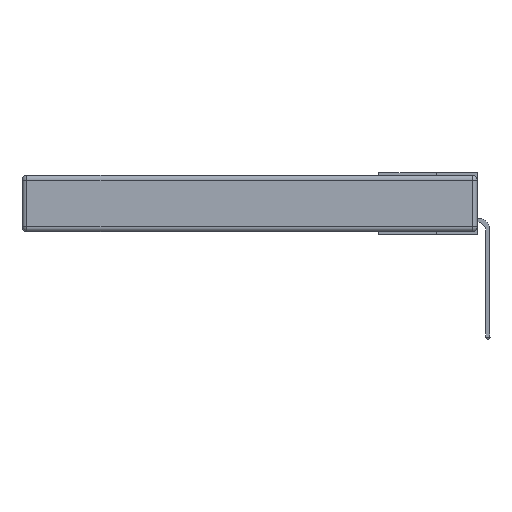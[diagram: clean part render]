
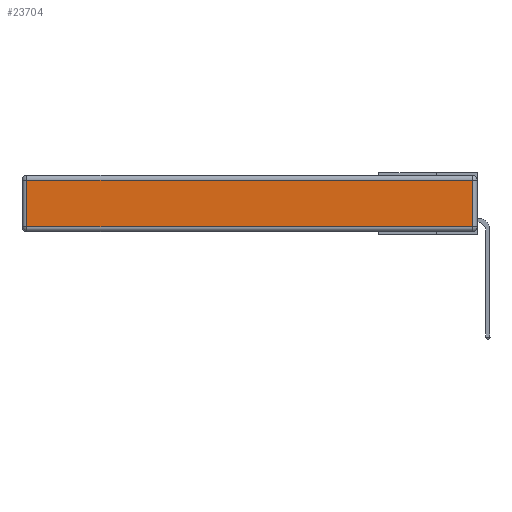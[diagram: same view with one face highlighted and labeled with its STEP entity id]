
A CAD part, left-side view. The second image highlights one B-rep face of the part: STEP entity #23704.
In plain terms, the highlighted planar face has unit normal (-1, 0, 0).
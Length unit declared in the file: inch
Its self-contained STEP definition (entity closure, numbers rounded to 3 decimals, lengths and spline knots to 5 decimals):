
#1822 = DIRECTION ( 'NONE',  ( 0., 0., 1. ) ) ;
#2178 = CARTESIAN_POINT ( 'NONE',  ( 0., 2.75, -0.03 ) ) ;
#3107 = CARTESIAN_POINT ( 'NONE',  ( 0., 0., -0.313 ) ) ;
#3621 = CARTESIAN_POINT ( 'NONE',  ( 0., 0.03, -0.343 ) ) ;
#4178 = LINE ( 'NONE', #2178, #25441 ) ;
#5476 = EDGE_CURVE ( 'NONE', #6696, #23846, #22380, .T. ) ;
#5622 = CARTESIAN_POINT ( 'NONE',  ( 0., 2.72, -0.313 ) ) ;
#6138 = VECTOR ( 'NONE', #21694, 39.37008 ) ;
#6536 = EDGE_CURVE ( 'NONE', #8301, #6696, #11588, .T. ) ;
#6542 = DIRECTION ( 'NONE',  ( 0., 0., -1. ) ) ;
#6696 = VERTEX_POINT ( 'NONE', #26419 ) ;
#6721 = CARTESIAN_POINT ( 'NONE',  ( 0., 2.72, -0.343 ) ) ;
#8301 = VERTEX_POINT ( 'NONE', #5622 ) ;
#9284 = VERTEX_POINT ( 'NONE', #10467 ) ;
#10467 = CARTESIAN_POINT ( 'NONE',  ( 0., 2.72, -0.03 ) ) ;
#11588 = LINE ( 'NONE', #3107, #6138 ) ;
#11650 = ORIENTED_EDGE ( 'NONE', *, *, #16790, .T. ) ;
#12256 = DIRECTION ( 'NONE',  ( 0., 1., 0. ) ) ;
#12745 = FACE_OUTER_BOUND ( 'NONE', #26552, .T. ) ;
#14138 = CARTESIAN_POINT ( 'NONE',  ( 0., 0., -0.343 ) ) ;
#14238 = DIRECTION ( 'NONE',  ( -1., 0., 0. ) ) ;
#14304 = VECTOR ( 'NONE', #6542, 39.37008 ) ;
#14691 = CARTESIAN_POINT ( 'NONE',  ( 0., 0.03, -0.03 ) ) ;
#16598 = LINE ( 'NONE', #6721, #14304 ) ;
#16790 = EDGE_CURVE ( 'NONE', #9284, #8301, #16598, .T. ) ;
#19874 = ORIENTED_EDGE ( 'NONE', *, *, #5476, .T. ) ;
#21694 = DIRECTION ( 'NONE',  ( 0., -1., 0. ) ) ;
#22050 = AXIS2_PLACEMENT_3D ( 'NONE', #14138, #14238, #1822 ) ;
#22304 = DIRECTION ( 'NONE',  ( 0., 0., 1. ) ) ;
#22380 = LINE ( 'NONE', #3621, #23644 ) ;
#22420 = EDGE_CURVE ( 'NONE', #23846, #9284, #4178, .T. ) ;
#23644 = VECTOR ( 'NONE', #22304, 39.37008 ) ;
#23704 = ADVANCED_FACE ( 'NONE', ( #12745 ), #24467, .T. ) ;
#23846 = VERTEX_POINT ( 'NONE', #14691 ) ;
#24467 = PLANE ( 'NONE',  #22050 ) ;
#25441 = VECTOR ( 'NONE', #12256, 39.37008 ) ;
#25622 = ORIENTED_EDGE ( 'NONE', *, *, #22420, .T. ) ;
#25872 = ORIENTED_EDGE ( 'NONE', *, *, #6536, .T. ) ;
#26419 = CARTESIAN_POINT ( 'NONE',  ( 0., 0.03, -0.313 ) ) ;
#26552 = EDGE_LOOP ( 'NONE', ( #25872, #19874, #25622, #11650 ) ) ;
